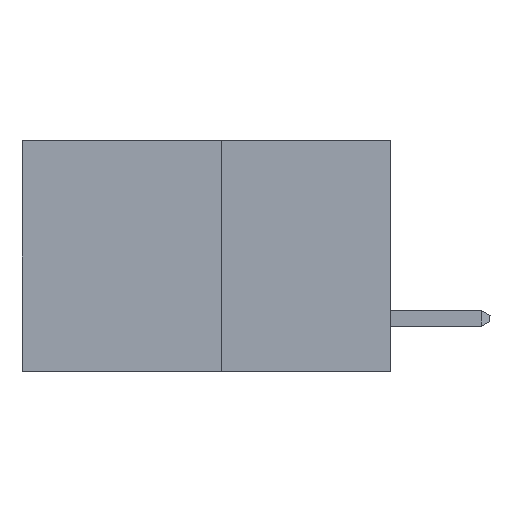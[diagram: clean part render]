
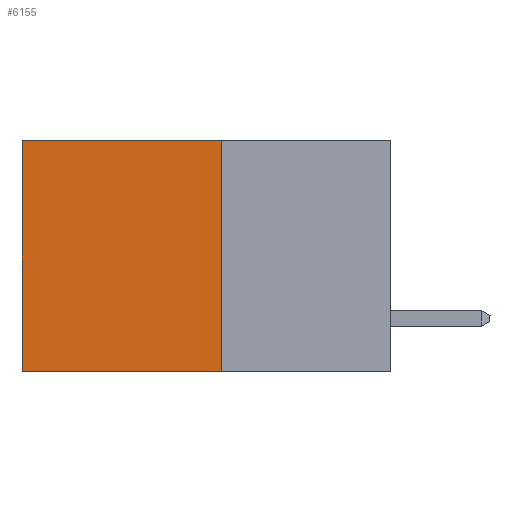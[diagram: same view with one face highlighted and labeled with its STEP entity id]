
A CAD part, left-side view. The second image highlights one B-rep face of the part: STEP entity #6155.
In plain terms, the highlighted planar face has unit normal (-1, 0, 0).
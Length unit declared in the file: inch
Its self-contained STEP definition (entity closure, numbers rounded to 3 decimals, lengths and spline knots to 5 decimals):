
#1390 = ORIENTED_EDGE ( 'NONE', *, *, #20222, .F. ) ;
#1784 = VERTEX_POINT ( 'NONE', #17798 ) ;
#2002 = DIRECTION ( 'NONE',  ( 0., 1., 0. ) ) ;
#3347 = ORIENTED_EDGE ( 'NONE', *, *, #5220, .T. ) ;
#3715 = AXIS2_PLACEMENT_3D ( 'NONE', #9623, #9558, #9493 ) ;
#4186 = DIRECTION ( 'NONE',  ( 0., 0., -1. ) ) ;
#5000 = LINE ( 'NONE', #13185, #13447 ) ;
#5152 = DIRECTION ( 'NONE',  ( 0., 0., -1. ) ) ;
#5220 = EDGE_CURVE ( 'NONE', #10112, #12969, #17586, .T. ) ;
#6104 = CARTESIAN_POINT ( 'NONE',  ( 0.277, 0.59, -0.37 ) ) ;
#6155 = ADVANCED_FACE ( 'NONE', ( #12939 ), #9743, .F. ) ;
#6734 = CARTESIAN_POINT ( 'NONE',  ( 0.277, 0.59, 0. ) ) ;
#8777 = ORIENTED_EDGE ( 'NONE', *, *, #9694, .F. ) ;
#9493 = DIRECTION ( 'NONE',  ( 0., 0., -1. ) ) ;
#9558 = DIRECTION ( 'NONE',  ( 1., 0., 0. ) ) ;
#9623 = CARTESIAN_POINT ( 'NONE',  ( 0.277, 0.27, -0.37 ) ) ;
#9694 = EDGE_CURVE ( 'NONE', #12524, #1784, #18246, .T. ) ;
#9743 = PLANE ( 'NONE',  #3715 ) ;
#10112 = VERTEX_POINT ( 'NONE', #6734 ) ;
#10352 = DIRECTION ( 'NONE',  ( 0., 1., 0. ) ) ;
#10452 = VECTOR ( 'NONE', #4186, 39.37008 ) ;
#12002 = CARTESIAN_POINT ( 'NONE',  ( 0.277, 0.59, -0.37 ) ) ;
#12524 = VERTEX_POINT ( 'NONE', #18584 ) ;
#12939 = FACE_OUTER_BOUND ( 'NONE', #15448, .T. ) ;
#12969 = VERTEX_POINT ( 'NONE', #12002 ) ;
#13185 = CARTESIAN_POINT ( 'NONE',  ( 0.277, 0.27, 0. ) ) ;
#13447 = VECTOR ( 'NONE', #2002, 39.37008 ) ;
#13460 = VECTOR ( 'NONE', #5152, 39.37008 ) ;
#13519 = CARTESIAN_POINT ( 'NONE',  ( 0.277, 0.27, -0.37 ) ) ;
#13691 = VECTOR ( 'NONE', #10352, 39.37008 ) ;
#13715 = CARTESIAN_POINT ( 'NONE',  ( 0.277, 0.27, -0.37 ) ) ;
#14644 = ORIENTED_EDGE ( 'NONE', *, *, #20059, .T. ) ;
#15448 = EDGE_LOOP ( 'NONE', ( #3347, #1390, #8777, #14644 ) ) ;
#17586 = LINE ( 'NONE', #6104, #13460 ) ;
#17798 = CARTESIAN_POINT ( 'NONE',  ( 0.277, 0.27, -0.37 ) ) ;
#17812 = LINE ( 'NONE', #13519, #13691 ) ;
#18246 = LINE ( 'NONE', #13715, #10452 ) ;
#18584 = CARTESIAN_POINT ( 'NONE',  ( 0.277, 0.27, 0. ) ) ;
#20059 = EDGE_CURVE ( 'NONE', #12524, #10112, #5000, .T. ) ;
#20222 = EDGE_CURVE ( 'NONE', #1784, #12969, #17812, .T. ) ;
